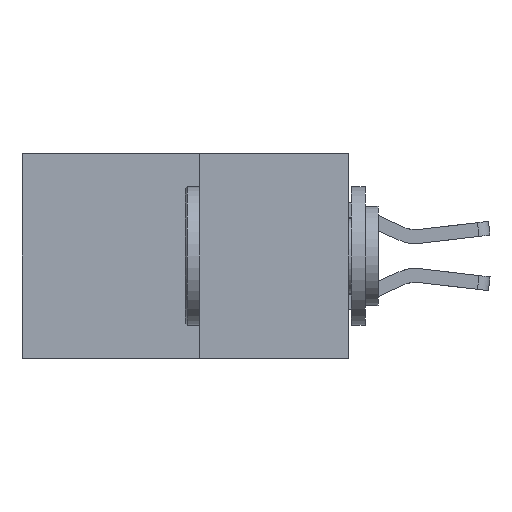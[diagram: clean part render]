
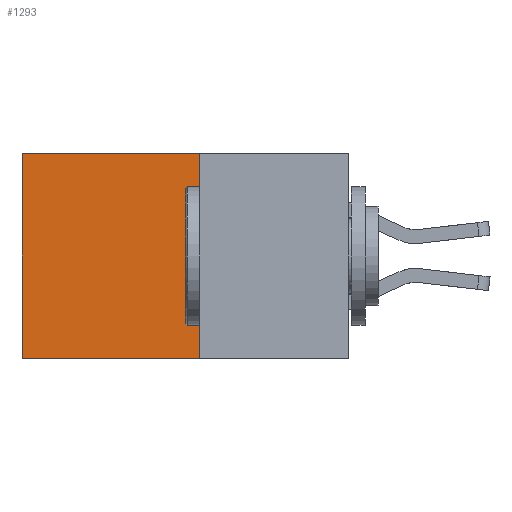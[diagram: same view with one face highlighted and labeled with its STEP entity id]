
A CAD part, left-side view. The second image highlights one B-rep face of the part: STEP entity #1293.
In plain terms, the highlighted planar face has unit normal (-1, 0, 0).
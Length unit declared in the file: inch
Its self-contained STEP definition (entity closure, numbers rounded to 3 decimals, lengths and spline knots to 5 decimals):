
#150 = AXIS2_PLACEMENT_3D ( 'NONE', #9547, #10200, #4982 ) ;
#519 = EDGE_CURVE ( 'NONE', #8552, #3671, #1846, .T. ) ;
#1122 = CARTESIAN_POINT ( 'NONE',  ( 0.277, 0.59, -0.37 ) ) ;
#1293 = ADVANCED_FACE ( 'NONE', ( #6837 ), #9432, .F. ) ;
#1321 = VECTOR ( 'NONE', #5853, 39.37008 ) ;
#1532 = VECTOR ( 'NONE', #5903, 39.37008 ) ;
#1794 = VERTEX_POINT ( 'NONE', #10752 ) ;
#1846 = LINE ( 'NONE', #4324, #1532 ) ;
#1885 = CARTESIAN_POINT ( 'NONE',  ( 0.277, 0.27, 0. ) ) ;
#1904 = CARTESIAN_POINT ( 'NONE',  ( 0.277, 0.59, -0.37 ) ) ;
#1996 = ORIENTED_EDGE ( 'NONE', *, *, #2059, .F. ) ;
#2059 = EDGE_CURVE ( 'NONE', #8552, #1794, #6155, .T. ) ;
#2256 = CARTESIAN_POINT ( 'NONE',  ( 0.277, 0.27, -0.37 ) ) ;
#2921 = EDGE_LOOP ( 'NONE', ( #7937, #10721, #1996, #9029 ) ) ;
#3671 = VERTEX_POINT ( 'NONE', #5137 ) ;
#4324 = CARTESIAN_POINT ( 'NONE',  ( 0.277, 0.27, 0. ) ) ;
#4982 = DIRECTION ( 'NONE',  ( 0., 0., -1. ) ) ;
#5137 = CARTESIAN_POINT ( 'NONE',  ( 0.277, 0.59, 0. ) ) ;
#5790 = CARTESIAN_POINT ( 'NONE',  ( 0.277, 0.27, -0.37 ) ) ;
#5853 = DIRECTION ( 'NONE',  ( 0., 0., -1. ) ) ;
#5903 = DIRECTION ( 'NONE',  ( 0., 1., 0. ) ) ;
#6155 = LINE ( 'NONE', #5790, #1321 ) ;
#6549 = DIRECTION ( 'NONE',  ( 0., 0., -1. ) ) ;
#6674 = VECTOR ( 'NONE', #6549, 39.37008 ) ;
#6837 = FACE_OUTER_BOUND ( 'NONE', #2921, .T. ) ;
#7282 = EDGE_CURVE ( 'NONE', #3671, #10227, #8982, .T. ) ;
#7359 = EDGE_CURVE ( 'NONE', #1794, #10227, #8160, .T. ) ;
#7937 = ORIENTED_EDGE ( 'NONE', *, *, #7282, .T. ) ;
#8160 = LINE ( 'NONE', #2256, #10679 ) ;
#8396 = DIRECTION ( 'NONE',  ( 0., 1., 0. ) ) ;
#8552 = VERTEX_POINT ( 'NONE', #1885 ) ;
#8982 = LINE ( 'NONE', #1122, #6674 ) ;
#9029 = ORIENTED_EDGE ( 'NONE', *, *, #519, .T. ) ;
#9432 = PLANE ( 'NONE',  #150 ) ;
#9547 = CARTESIAN_POINT ( 'NONE',  ( 0.277, 0.27, -0.37 ) ) ;
#10200 = DIRECTION ( 'NONE',  ( 1., 0., 0. ) ) ;
#10227 = VERTEX_POINT ( 'NONE', #1904 ) ;
#10679 = VECTOR ( 'NONE', #8396, 39.37008 ) ;
#10721 = ORIENTED_EDGE ( 'NONE', *, *, #7359, .F. ) ;
#10752 = CARTESIAN_POINT ( 'NONE',  ( 0.277, 0.27, -0.37 ) ) ;
